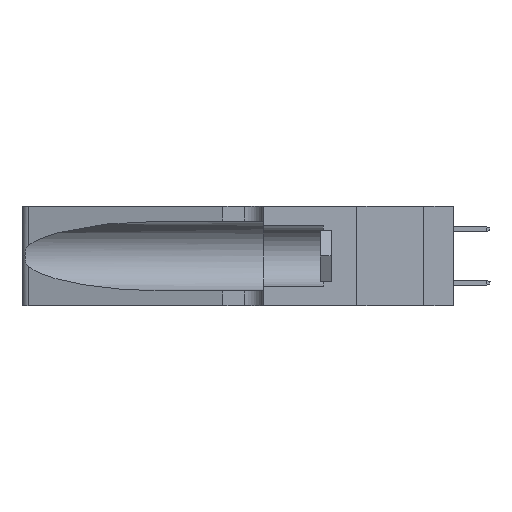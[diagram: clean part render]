
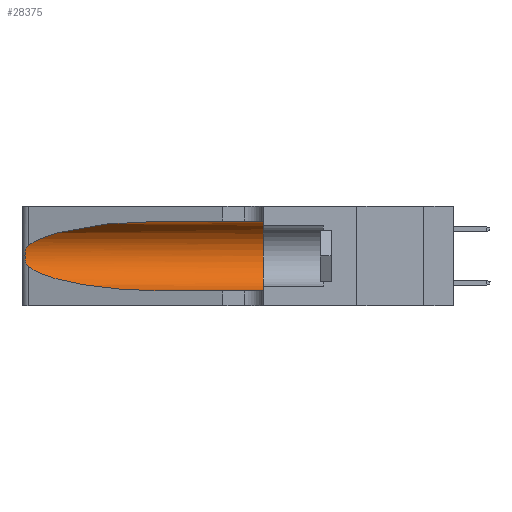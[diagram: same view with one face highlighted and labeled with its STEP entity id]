
A CAD part, left-side view. The second image highlights one B-rep face of the part: STEP entity #28375.
In plain terms, the highlighted cylindrical face has radius 3.308 mm (diameter 6.617 mm), a partial arc.
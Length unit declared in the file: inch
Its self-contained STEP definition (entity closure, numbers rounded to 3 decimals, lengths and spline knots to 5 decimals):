
#306 = CARTESIAN_POINT ( 'NONE',  ( 0.1305, 0.35, 0.05475 ) ) ;
#611 = CARTESIAN_POINT ( 'NONE',  ( 0.2373, 1.15595, 0.28018 ) ) ;
#1002 = CARTESIAN_POINT ( 'NONE',  ( 0.26075, 1.23896, 0.178 ) ) ;
#3028 = CARTESIAN_POINT ( 'NONE',  ( 0.1305, 0.72297, 0.31525 ) ) ;
#3564 = EDGE_CURVE ( 'NONE', #17287, #15864, #38329, .T. ) ;
#4009 = DIRECTION ( 'NONE',  ( 0., 1., 0. ) ) ;
#5340 = LINE ( 'NONE', #5546, #5650 ) ;
#5546 = CARTESIAN_POINT ( 'NONE',  ( 0.1305, 1.61858, 0.05475 ) ) ;
#5648 = AXIS2_PLACEMENT_3D ( 'NONE', #22757, #29055, #34522 ) ;
#5650 = VECTOR ( 'NONE', #13830, 39.37008 ) ;
#6671 = CARTESIAN_POINT ( 'NONE',  ( 0.25487, 1.22718, 0.22369 ) ) ;
#7201 = ORIENTED_EDGE ( 'NONE', *, *, #13002, .F. ) ;
#10494 = FACE_OUTER_BOUND ( 'NONE', #19773, .T. ) ;
#11105 = VERTEX_POINT ( 'NONE', #37015 ) ;
#11427 = CARTESIAN_POINT ( 'NONE',  ( 0.1305, 0.72297, 0.05475 ) ) ;
#12411 = VERTEX_POINT ( 'NONE', #21963 ) ;
#12803 = ORIENTED_EDGE ( 'NONE', *, *, #16020, .T. ) ;
#12911 = CARTESIAN_POINT ( 'NONE',  ( 0.25639, 1.23184, 0.21858 ) ) ;
#13002 = EDGE_CURVE ( 'NONE', #19435, #17287, #23063, .T. ) ;
#13309 = CARTESIAN_POINT ( 'NONE',  ( 0.25856, 1.23593, 0.16098 ) ) ;
#13314 = CARTESIAN_POINT ( 'NONE',  ( 0.18966, 0.96281, 0.31525 ) ) ;
#13830 = DIRECTION ( 'NONE',  ( 0., -1., 0. ) ) ;
#14509 = ORIENTED_EDGE ( 'NONE', *, *, #28184, .T. ) ;
#15864 = VERTEX_POINT ( 'NONE', #306 ) ;
#16020 = EDGE_CURVE ( 'NONE', #19435, #11105, #31496, .T. ) ;
#16320 = DIRECTION ( 'NONE',  ( 0., 0., 1. ) ) ;
#16338 = CARTESIAN_POINT ( 'NONE',  ( 0.25854, 1.2359, 0.20912 ) ) ;
#17000 = VERTEX_POINT ( 'NONE', #11427 ) ;
#17287 = VERTEX_POINT ( 'NONE', #23216 ) ;
#19333 = B_SPLINE_CURVE_WITH_KNOTS ( 'NONE', 3,
 ( #19352, #22565, #12911, #22178, #16338, #28661, #34525, #1002, #31882, #13309, #25600, #37966, #28862, #19943 ),
 .UNSPECIFIED., .F., .F.,
 ( 4, 2, 2, 2, 2, 2, 4 ),
 ( 0., 0.00027, 0.00053, 0.00107, 0.0016, 0.00187, 0.00214 ),
 .UNSPECIFIED. ) ;
#19352 = CARTESIAN_POINT ( 'NONE',  ( 0.25487, 1.22718, 0.22369 ) ) ;
#19435 = VERTEX_POINT ( 'NONE', #3028 ) ;
#19555 = CYLINDRICAL_SURFACE ( 'NONE', #5648, 0.13025 ) ;
#19773 = EDGE_LOOP ( 'NONE', ( #12803, #23650, #14509, #23684, #26644, #7201 ) ) ;
#19943 = CARTESIAN_POINT ( 'NONE',  ( 0.25487, 1.22718, 0.14631 ) ) ;
#21768 = CARTESIAN_POINT ( 'NONE',  ( 0.18966, 0.96281, 0.05475 ) ) ;
#21963 = CARTESIAN_POINT ( 'NONE',  ( 0.25487, 1.22718, 0.14631 ) ) ;
#22178 = CARTESIAN_POINT ( 'NONE',  ( 0.25787, 1.23484, 0.2124 ) ) ;
#22565 = CARTESIAN_POINT ( 'NONE',  ( 0.25555, 1.22994, 0.2215 ) ) ;
#22757 = CARTESIAN_POINT ( 'NONE',  ( 0.1305, 1.61858, 0.185 ) ) ;
#23063 = LINE ( 'NONE', #29559, #36243 ) ;
#23216 = CARTESIAN_POINT ( 'NONE',  ( 0.1305, 0.35, 0.31525 ) ) ;
#23650 = ORIENTED_EDGE ( 'NONE', *, *, #33645, .T. ) ;
#23684 = ORIENTED_EDGE ( 'NONE', *, *, #27130, .T. ) ;
#25205 = CARTESIAN_POINT ( 'NONE',  ( 0.1305, 0.72297, 0.31525 ) ) ;
#25600 = CARTESIAN_POINT ( 'NONE',  ( 0.25789, 1.23486, 0.15765 ) ) ;
#26644 = ORIENTED_EDGE ( 'NONE', *, *, #3564, .F. ) ;
#27130 = EDGE_CURVE ( 'NONE', #17000, #15864, #5340, .T. ) ;
#28057 = CARTESIAN_POINT ( 'NONE',  ( 0.25487, 1.22718, 0.14631 ) ) ;
#28184 = EDGE_CURVE ( 'NONE', #12411, #17000, #35889, .T. ) ;
#28375 = ADVANCED_FACE ( 'NONE', ( #10494 ), #19555, .F. ) ;
#28615 = AXIS2_PLACEMENT_3D ( 'NONE', #31656, #4009, #16320 ) ;
#28661 = CARTESIAN_POINT ( 'NONE',  ( 0.26018, 1.23835, 0.19895 ) ) ;
#28862 = CARTESIAN_POINT ( 'NONE',  ( 0.25555, 1.22993, 0.14849 ) ) ;
#29055 = DIRECTION ( 'NONE',  ( 0., -1., 0. ) ) ;
#29559 = CARTESIAN_POINT ( 'NONE',  ( 0.1305, 1.61858, 0.31525 ) ) ;
#31496 =( BOUNDED_CURVE ( )  B_SPLINE_CURVE ( 3, ( #25205, #13314, #611, #6671 ),
 .UNSPECIFIED., .F., .F. ) 
 B_SPLINE_CURVE_WITH_KNOTS ( ( 4, 4 ),
 ( 1.5708, 2.84003 ),
 .UNSPECIFIED. ) 
 CURVE ( )  GEOMETRIC_REPRESENTATION_ITEM ( )  RATIONAL_B_SPLINE_CURVE ( ( 1., 0.87, 0.87, 1. ) ) 
 REPRESENTATION_ITEM ( '' )  );
#31656 = CARTESIAN_POINT ( 'NONE',  ( 0.1305, 0.35, 0.185 ) ) ;
#31882 = CARTESIAN_POINT ( 'NONE',  ( 0.26017, 1.23833, 0.17102 ) ) ;
#33645 = EDGE_CURVE ( 'NONE', #11105, #12411, #19333, .T. ) ;
#33721 = CARTESIAN_POINT ( 'NONE',  ( 0.2373, 1.15595, 0.08982 ) ) ;
#34522 = DIRECTION ( 'NONE',  ( 0., 0., -1. ) ) ;
#34525 = CARTESIAN_POINT ( 'NONE',  ( 0.26075, 1.23896, 0.19203 ) ) ;
#35229 = DIRECTION ( 'NONE',  ( 0., -1., 0. ) ) ;
#35889 =( BOUNDED_CURVE ( )  B_SPLINE_CURVE ( 3, ( #28057, #33721, #21768, #36958 ),
 .UNSPECIFIED., .F., .F. ) 
 B_SPLINE_CURVE_WITH_KNOTS ( ( 4, 4 ),
 ( 3.44316, 4.71239 ),
 .UNSPECIFIED. ) 
 CURVE ( )  GEOMETRIC_REPRESENTATION_ITEM ( )  RATIONAL_B_SPLINE_CURVE ( ( 1., 0.87, 0.87, 1. ) ) 
 REPRESENTATION_ITEM ( '' )  );
#36243 = VECTOR ( 'NONE', #35229, 39.37008 ) ;
#36958 = CARTESIAN_POINT ( 'NONE',  ( 0.1305, 0.72297, 0.05475 ) ) ;
#37015 = CARTESIAN_POINT ( 'NONE',  ( 0.25487, 1.22718, 0.22369 ) ) ;
#37966 = CARTESIAN_POINT ( 'NONE',  ( 0.25639, 1.23186, 0.15144 ) ) ;
#38329 = CIRCLE ( 'NONE', #28615, 0.13025 ) ;
